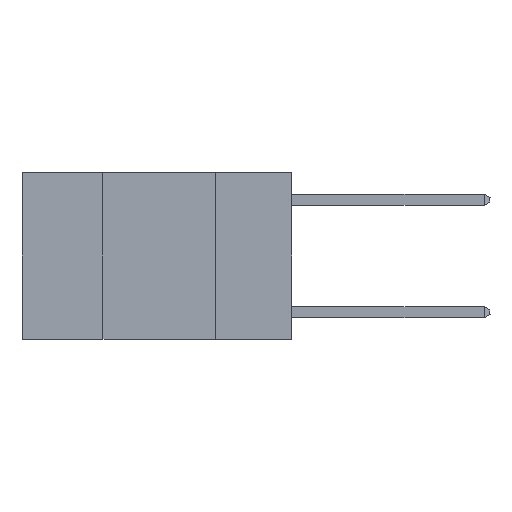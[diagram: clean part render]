
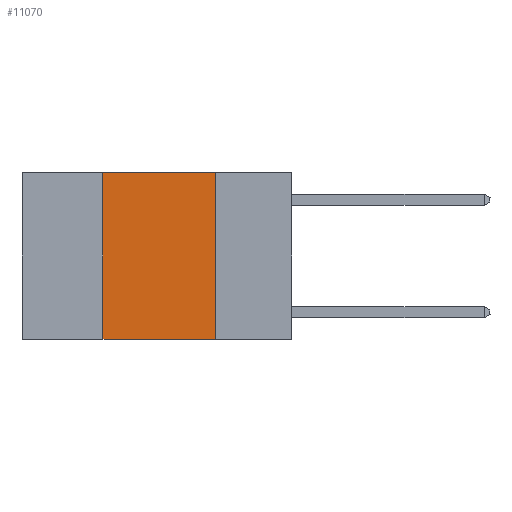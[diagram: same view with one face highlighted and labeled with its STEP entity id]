
A CAD part, left-side view. The second image highlights one B-rep face of the part: STEP entity #11070.
In plain terms, the highlighted planar face has unit normal (-1, 0, 0).
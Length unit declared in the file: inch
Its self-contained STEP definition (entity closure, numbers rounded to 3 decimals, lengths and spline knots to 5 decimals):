
#380 = CARTESIAN_POINT ( 'NONE',  ( 0., 0.42, 0. ) ) ;
#1040 = DIRECTION ( 'NONE',  ( 0., 0., -1. ) ) ;
#1053 = VERTEX_POINT ( 'NONE', #15905 ) ;
#1443 = CARTESIAN_POINT ( 'NONE',  ( 0., 0.6, 0. ) ) ;
#2458 = CARTESIAN_POINT ( 'NONE',  ( 0., 0.17, 0. ) ) ;
#2541 = EDGE_CURVE ( 'NONE', #20214, #18251, #19283, .T. ) ;
#2961 = DIRECTION ( 'NONE',  ( 0., -1., 0. ) ) ;
#3199 = AXIS2_PLACEMENT_3D ( 'NONE', #1443, #8034, #1040 ) ;
#3243 = EDGE_CURVE ( 'NONE', #15810, #20214, #20493, .T. ) ;
#5355 = ORIENTED_EDGE ( 'NONE', *, *, #3243, .F. ) ;
#5385 = VECTOR ( 'NONE', #14037, 39.37008 ) ;
#5721 = VECTOR ( 'NONE', #7182, 39.37008 ) ;
#6043 = VECTOR ( 'NONE', #17663, 39.37008 ) ;
#6202 = CARTESIAN_POINT ( 'NONE',  ( 0., 0.6, -0.37 ) ) ;
#6224 = CARTESIAN_POINT ( 'NONE',  ( 0., 0.17, -0.37 ) ) ;
#7030 = ORIENTED_EDGE ( 'NONE', *, *, #2541, .F. ) ;
#7182 = DIRECTION ( 'NONE',  ( 0., 0., 1. ) ) ;
#7261 = ORIENTED_EDGE ( 'NONE', *, *, #15583, .F. ) ;
#8034 = DIRECTION ( 'NONE',  ( 1., 0., 0. ) ) ;
#9230 = ORIENTED_EDGE ( 'NONE', *, *, #18748, .T. ) ;
#9658 = PLANE ( 'NONE',  #3199 ) ;
#11070 = ADVANCED_FACE ( 'NONE', ( #15809 ), #9658, .F. ) ;
#14027 = VECTOR ( 'NONE', #2961, 39.37008 ) ;
#14037 = DIRECTION ( 'NONE',  ( 0., -1., 0. ) ) ;
#14844 = EDGE_LOOP ( 'NONE', ( #7030, #5355, #7261, #9230 ) ) ;
#15006 = CARTESIAN_POINT ( 'NONE',  ( 0., 0.42, 0. ) ) ;
#15583 = EDGE_CURVE ( 'NONE', #1053, #15810, #18709, .T. ) ;
#15809 = FACE_OUTER_BOUND ( 'NONE', #14844, .T. ) ;
#15810 = VERTEX_POINT ( 'NONE', #15006 ) ;
#15905 = CARTESIAN_POINT ( 'NONE',  ( 0., 0.42, -0.37 ) ) ;
#17663 = DIRECTION ( 'NONE',  ( 0., 0., -1. ) ) ;
#18251 = VERTEX_POINT ( 'NONE', #6224 ) ;
#18683 = CARTESIAN_POINT ( 'NONE',  ( 0., 0.6, 0. ) ) ;
#18709 = LINE ( 'NONE', #380, #5721 ) ;
#18748 = EDGE_CURVE ( 'NONE', #1053, #18251, #20990, .T. ) ;
#19283 = LINE ( 'NONE', #2458, #6043 ) ;
#19972 = CARTESIAN_POINT ( 'NONE',  ( 0., 0.17, 0. ) ) ;
#20214 = VERTEX_POINT ( 'NONE', #19972 ) ;
#20493 = LINE ( 'NONE', #18683, #5385 ) ;
#20990 = LINE ( 'NONE', #6202, #14027 ) ;
